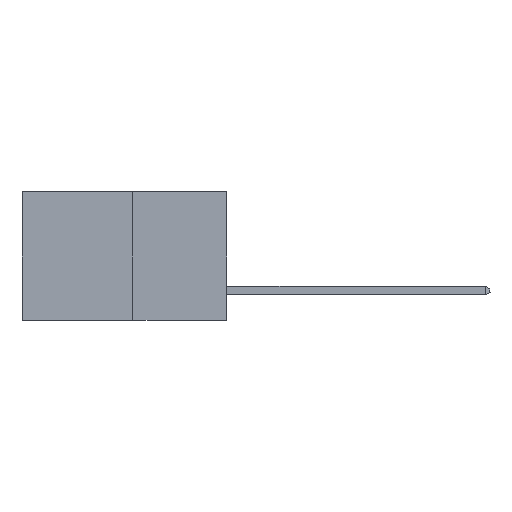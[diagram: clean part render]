
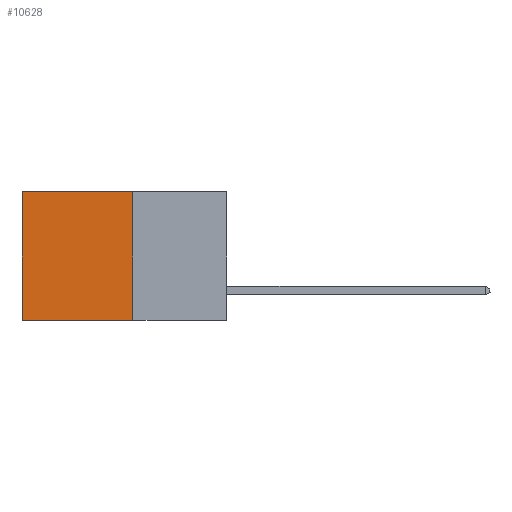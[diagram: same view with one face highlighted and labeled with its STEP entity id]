
A CAD part, left-side view. The second image highlights one B-rep face of the part: STEP entity #10628.
In plain terms, the highlighted planar face has unit normal (-1, 0, 0).
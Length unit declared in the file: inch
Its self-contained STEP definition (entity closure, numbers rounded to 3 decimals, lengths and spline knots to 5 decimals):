
#48 = ORIENTED_EDGE ( 'NONE', *, *, #8550, .T. ) ;
#110 = ORIENTED_EDGE ( 'NONE', *, *, #10853, .F. ) ;
#484 = ORIENTED_EDGE ( 'NONE', *, *, #10430, .F. ) ;
#612 = DIRECTION ( 'NONE',  ( 0., 0., -1. ) ) ;
#736 = LINE ( 'NONE', #12655, #11976 ) ;
#839 = ORIENTED_EDGE ( 'NONE', *, *, #4044, .T. ) ;
#1299 = VERTEX_POINT ( 'NONE', #12258 ) ;
#1409 = DIRECTION ( 'NONE',  ( 0., 0., -1. ) ) ;
#1478 = FACE_OUTER_BOUND ( 'NONE', #8041, .T. ) ;
#2855 = VECTOR ( 'NONE', #1409, 39.37008 ) ;
#3005 = CARTESIAN_POINT ( 'NONE',  ( 0.277, 0.27, -0.37 ) ) ;
#3253 = CARTESIAN_POINT ( 'NONE',  ( 0.277, 0.27, -0.37 ) ) ;
#3320 = CARTESIAN_POINT ( 'NONE',  ( 0.277, 0.59, -0.37 ) ) ;
#4044 = EDGE_CURVE ( 'NONE', #4419, #1299, #736, .T. ) ;
#4419 = VERTEX_POINT ( 'NONE', #6438 ) ;
#5985 = VECTOR ( 'NONE', #612, 39.37008 ) ;
#6407 = PLANE ( 'NONE',  #9722 ) ;
#6438 = CARTESIAN_POINT ( 'NONE',  ( 0.277, 0.27, 0. ) ) ;
#7451 = DIRECTION ( 'NONE',  ( 0., 0., -1. ) ) ;
#7888 = VERTEX_POINT ( 'NONE', #3253 ) ;
#8041 = EDGE_LOOP ( 'NONE', ( #48, #110, #484, #839 ) ) ;
#8366 = CARTESIAN_POINT ( 'NONE',  ( 0.277, 0.59, -0.37 ) ) ;
#8502 = LINE ( 'NONE', #8366, #5985 ) ;
#8550 = EDGE_CURVE ( 'NONE', #1299, #11386, #8502, .T. ) ;
#8772 = CARTESIAN_POINT ( 'NONE',  ( 0.277, 0.27, -0.37 ) ) ;
#9071 = LINE ( 'NONE', #9133, #2855 ) ;
#9133 = CARTESIAN_POINT ( 'NONE',  ( 0.277, 0.27, -0.37 ) ) ;
#9722 = AXIS2_PLACEMENT_3D ( 'NONE', #3005, #13570, #7451 ) ;
#10430 = EDGE_CURVE ( 'NONE', #4419, #7888, #9071, .T. ) ;
#10628 = ADVANCED_FACE ( 'NONE', ( #1478 ), #6407, .F. ) ;
#10853 = EDGE_CURVE ( 'NONE', #7888, #11386, #13730, .T. ) ;
#11237 = VECTOR ( 'NONE', #12887, 39.37008 ) ;
#11386 = VERTEX_POINT ( 'NONE', #3320 ) ;
#11976 = VECTOR ( 'NONE', #12527, 39.37008 ) ;
#12258 = CARTESIAN_POINT ( 'NONE',  ( 0.277, 0.59, 0. ) ) ;
#12527 = DIRECTION ( 'NONE',  ( 0., 1., 0. ) ) ;
#12655 = CARTESIAN_POINT ( 'NONE',  ( 0.277, 0.27, 0. ) ) ;
#12887 = DIRECTION ( 'NONE',  ( 0., 1., 0. ) ) ;
#13570 = DIRECTION ( 'NONE',  ( 1., 0., 0. ) ) ;
#13730 = LINE ( 'NONE', #8772, #11237 ) ;
